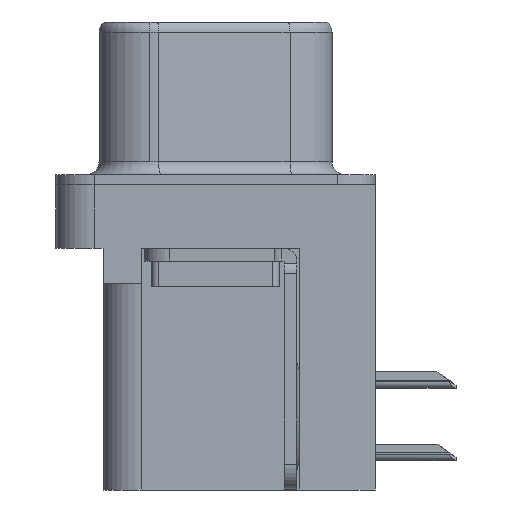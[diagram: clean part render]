
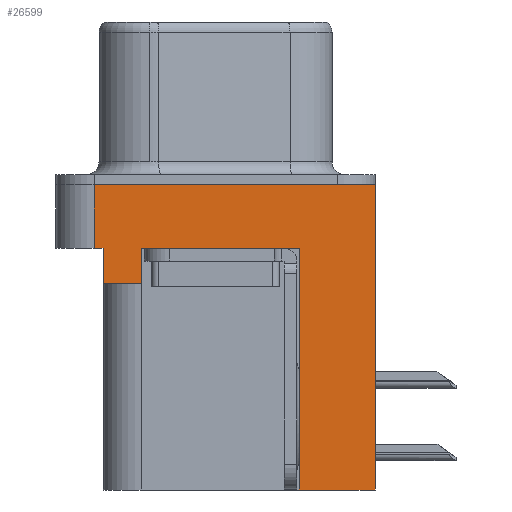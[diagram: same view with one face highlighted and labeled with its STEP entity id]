
A CAD part, left-side view. The second image highlights one B-rep face of the part: STEP entity #26599.
In plain terms, the highlighted planar face has unit normal (-1, 0, 0).
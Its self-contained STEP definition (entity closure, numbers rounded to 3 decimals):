
#34 = VERTEX_POINT ( 'NONE', #24204 ) ;
#721 = LINE ( 'NONE', #3891, #22890 ) ;
#2255 = EDGE_CURVE ( 'NONE', #5230, #23466, #22655, .T. ) ;
#2688 = VECTOR ( 'NONE', #16237, 1000. ) ;
#3074 = PLANE ( 'NONE',  #5514 ) ;
#3241 = ORIENTED_EDGE ( 'NONE', *, *, #4614, .F. ) ;
#3726 = EDGE_LOOP ( 'NONE', ( #22088, #23667, #18619, #3241, #25933, #17475, #11622, #16881, #20711, #17724 ) ) ;
#3891 = CARTESIAN_POINT ( 'NONE',  ( -2.91, -3.295, -12. ) ) ;
#3911 = CARTESIAN_POINT ( 'NONE',  ( -2.91, 4.425, -3.9 ) ) ;
#4310 = CARTESIAN_POINT ( 'NONE',  ( -2.91, 2.895, -3.9 ) ) ;
#4614 = EDGE_CURVE ( 'NONE', #14644, #17678, #14902, .T. ) ;
#4985 = VECTOR ( 'NONE', #22552, 1000. ) ;
#4999 = DIRECTION ( 'NONE',  ( -1., 0., 0. ) ) ;
#5230 = VERTEX_POINT ( 'NONE', #8681 ) ;
#5514 = AXIS2_PLACEMENT_3D ( 'NONE', #11810, #4999, #16131 ) ;
#6652 = EDGE_CURVE ( 'NONE', #27041, #14644, #18042, .T. ) ;
#7000 = LINE ( 'NONE', #13297, #24017 ) ;
#7047 = CARTESIAN_POINT ( 'NONE',  ( -2.91, 4.425, -3.9 ) ) ;
#7065 = LINE ( 'NONE', #28197, #19211 ) ;
#7457 = CARTESIAN_POINT ( 'NONE',  ( -2.91, -6.275, -2.5 ) ) ;
#7550 = DIRECTION ( 'NONE',  ( 0., 0., 1. ) ) ;
#8164 = EDGE_CURVE ( 'NONE', #27041, #20206, #21143, .T. ) ;
#8582 = EDGE_CURVE ( 'NONE', #18776, #14903, #721, .T. ) ;
#8681 = CARTESIAN_POINT ( 'NONE',  ( -2.91, 4.775, 0. ) ) ;
#8736 = EDGE_CURVE ( 'NONE', #18776, #23466, #22529, .T. ) ;
#10045 = VECTOR ( 'NONE', #14512, 1000. ) ;
#10417 = DIRECTION ( 'NONE',  ( 0., 0., 1. ) ) ;
#10984 = CARTESIAN_POINT ( 'NONE',  ( -2.91, -3.295, -2.5 ) ) ;
#11209 = CARTESIAN_POINT ( 'NONE',  ( -2.91, -6.275, -2.5 ) ) ;
#11622 = ORIENTED_EDGE ( 'NONE', *, *, #13773, .T. ) ;
#11810 = CARTESIAN_POINT ( 'NONE',  ( -2.91, -6.275, -2.5 ) ) ;
#12944 = DIRECTION ( 'NONE',  ( 0., 0., 1. ) ) ;
#13267 = EDGE_CURVE ( 'NONE', #34, #5230, #26896, .T. ) ;
#13297 = CARTESIAN_POINT ( 'NONE',  ( -2.91, -6.275, -2.5 ) ) ;
#13551 = CARTESIAN_POINT ( 'NONE',  ( -2.91, -3.295, -12. ) ) ;
#13773 = EDGE_CURVE ( 'NONE', #20206, #25671, #7000, .T. ) ;
#14512 = DIRECTION ( 'NONE',  ( 0., 1., 0. ) ) ;
#14560 = VECTOR ( 'NONE', #18081, 1000. ) ;
#14644 = VERTEX_POINT ( 'NONE', #22879 ) ;
#14902 = LINE ( 'NONE', #7047, #14560 ) ;
#14903 = VERTEX_POINT ( 'NONE', #13551 ) ;
#15307 = CARTESIAN_POINT ( 'NONE',  ( -2.91, 4.425, -2.5 ) ) ;
#15584 = DIRECTION ( 'NONE',  ( 0., -1., 0. ) ) ;
#16131 = DIRECTION ( 'NONE',  ( 0., 0., 1. ) ) ;
#16237 = DIRECTION ( 'NONE',  ( 0., 0., 1. ) ) ;
#16651 = VECTOR ( 'NONE', #7550, 1000. ) ;
#16881 = ORIENTED_EDGE ( 'NONE', *, *, #18708, .F. ) ;
#17472 = VECTOR ( 'NONE', #24787, 1000. ) ;
#17475 = ORIENTED_EDGE ( 'NONE', *, *, #8164, .T. ) ;
#17678 = VERTEX_POINT ( 'NONE', #15307 ) ;
#17724 = ORIENTED_EDGE ( 'NONE', *, *, #8736, .T. ) ;
#18042 = LINE ( 'NONE', #3911, #10045 ) ;
#18081 = DIRECTION ( 'NONE',  ( 0., 0., 1. ) ) ;
#18619 = ORIENTED_EDGE ( 'NONE', *, *, #21312, .T. ) ;
#18708 = EDGE_CURVE ( 'NONE', #14903, #25671, #7065, .T. ) ;
#18776 = VERTEX_POINT ( 'NONE', #21979 ) ;
#19211 = VECTOR ( 'NONE', #12944, 1000. ) ;
#19359 = DIRECTION ( 'NONE',  ( 0., 1., 0. ) ) ;
#20206 = VERTEX_POINT ( 'NONE', #27748 ) ;
#20246 = LINE ( 'NONE', #11209, #4985 ) ;
#20711 = ORIENTED_EDGE ( 'NONE', *, *, #8582, .F. ) ;
#21143 = LINE ( 'NONE', #22099, #28443 ) ;
#21312 = EDGE_CURVE ( 'NONE', #34, #17678, #20246, .T. ) ;
#21979 = CARTESIAN_POINT ( 'NONE',  ( -2.91, -6.275, -12. ) ) ;
#22088 = ORIENTED_EDGE ( 'NONE', *, *, #2255, .F. ) ;
#22099 = CARTESIAN_POINT ( 'NONE',  ( -2.91, 2.895, -3.9 ) ) ;
#22529 = LINE ( 'NONE', #7457, #16651 ) ;
#22552 = DIRECTION ( 'NONE',  ( 0., -1., 0. ) ) ;
#22568 = CARTESIAN_POINT ( 'NONE',  ( -2.91, -6.275, 0. ) ) ;
#22655 = LINE ( 'NONE', #22568, #17472 ) ;
#22713 = CARTESIAN_POINT ( 'NONE',  ( -2.91, 4.775, -2.5 ) ) ;
#22879 = CARTESIAN_POINT ( 'NONE',  ( -2.91, 4.425, -3.9 ) ) ;
#22890 = VECTOR ( 'NONE', #19359, 1000. ) ;
#23450 = CARTESIAN_POINT ( 'NONE',  ( -2.91, -6.275, 0. ) ) ;
#23466 = VERTEX_POINT ( 'NONE', #23450 ) ;
#23667 = ORIENTED_EDGE ( 'NONE', *, *, #13267, .F. ) ;
#24017 = VECTOR ( 'NONE', #15584, 1000. ) ;
#24204 = CARTESIAN_POINT ( 'NONE',  ( -2.91, 4.775, -2.5 ) ) ;
#24787 = DIRECTION ( 'NONE',  ( 0., -1., 0. ) ) ;
#25671 = VERTEX_POINT ( 'NONE', #10984 ) ;
#25933 = ORIENTED_EDGE ( 'NONE', *, *, #6652, .F. ) ;
#26551 = FACE_OUTER_BOUND ( 'NONE', #3726, .T. ) ;
#26599 = ADVANCED_FACE ( 'NONE', ( #26551 ), #3074, .T. ) ;
#26896 = LINE ( 'NONE', #22713, #2688 ) ;
#27041 = VERTEX_POINT ( 'NONE', #4310 ) ;
#27748 = CARTESIAN_POINT ( 'NONE',  ( -2.91, 2.895, -2.5 ) ) ;
#28197 = CARTESIAN_POINT ( 'NONE',  ( -2.91, -3.295, -12. ) ) ;
#28443 = VECTOR ( 'NONE', #10417, 1000. ) ;
